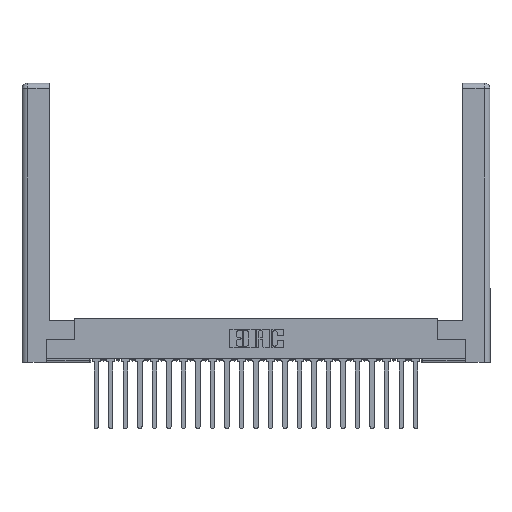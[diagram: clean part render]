
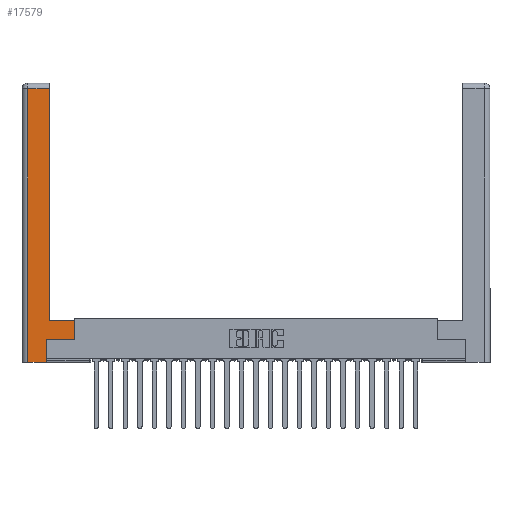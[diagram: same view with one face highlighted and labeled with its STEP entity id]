
A CAD part, top view. The second image highlights one B-rep face of the part: STEP entity #17579.
In plain terms, the highlighted planar face has unit normal (0, 0, 1).
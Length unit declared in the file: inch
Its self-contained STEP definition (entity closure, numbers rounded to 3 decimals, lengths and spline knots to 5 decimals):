
#313 = VERTEX_POINT ( 'NONE', #2295 ) ;
#631 = CARTESIAN_POINT ( 'NONE',  ( 0.265, 0.245, 0. ) ) ;
#657 = VERTEX_POINT ( 'NONE', #1518 ) ;
#1205 = CARTESIAN_POINT ( 'NONE',  ( 0.0615, 2.94, 0. ) ) ;
#1265 = EDGE_CURVE ( 'NONE', #10887, #19889, #2204, .T. ) ;
#1518 = CARTESIAN_POINT ( 'NONE',  ( 0.265, 0., 0. ) ) ;
#1738 = EDGE_CURVE ( 'NONE', #21075, #10887, #23400, .T. ) ;
#1778 = CARTESIAN_POINT ( 'NONE',  ( 0.295, 0.45, 0. ) ) ;
#2204 = LINE ( 'NONE', #16400, #24942 ) ;
#2295 = CARTESIAN_POINT ( 'NONE',  ( 0.265, 0.245, 0. ) ) ;
#2714 = CARTESIAN_POINT ( 'NONE',  ( 0.0615, 2.94, 0. ) ) ;
#4277 = FACE_OUTER_BOUND ( 'NONE', #4990, .T. ) ;
#4420 = ORIENTED_EDGE ( 'NONE', *, *, #1738, .T. ) ;
#4990 = EDGE_LOOP ( 'NONE', ( #19216, #16404, #6336, #10383, #8769, #19691, #4420, #19415 ) ) ;
#5322 = EDGE_CURVE ( 'NONE', #23541, #657, #14976, .T. ) ;
#5569 = CARTESIAN_POINT ( 'NONE',  ( 0.265, 0., 0. ) ) ;
#5839 = VERTEX_POINT ( 'NONE', #9261 ) ;
#5865 = VECTOR ( 'NONE', #8945, 39.37008 ) ;
#5916 = VECTOR ( 'NONE', #13817, 39.37008 ) ;
#6336 = ORIENTED_EDGE ( 'NONE', *, *, #19013, .T. ) ;
#6571 = DIRECTION ( 'NONE',  ( 0., -1., 0. ) ) ;
#7114 = DIRECTION ( 'NONE',  ( -1., 0., 0. ) ) ;
#7325 = LINE ( 'NONE', #16504, #15325 ) ;
#7489 = EDGE_CURVE ( 'NONE', #19889, #5839, #20387, .T. ) ;
#8356 = EDGE_CURVE ( 'NONE', #5839, #15024, #16033, .T. ) ;
#8667 = DIRECTION ( 'NONE',  ( -1., 0., 0. ) ) ;
#8769 = ORIENTED_EDGE ( 'NONE', *, *, #9873, .T. ) ;
#8945 = DIRECTION ( 'NONE',  ( 0., 1., 0. ) ) ;
#9261 = CARTESIAN_POINT ( 'NONE',  ( 0.295, 2.94, 0. ) ) ;
#9380 = DIRECTION ( 'NONE',  ( 1., 0., 0. ) ) ;
#9615 = VECTOR ( 'NONE', #7114, 39.37008 ) ;
#9733 = CARTESIAN_POINT ( 'NONE',  ( 0.0615, 0., 0. ) ) ;
#9873 = EDGE_CURVE ( 'NONE', #657, #313, #15981, .T. ) ;
#10383 = ORIENTED_EDGE ( 'NONE', *, *, #5322, .T. ) ;
#10887 = VERTEX_POINT ( 'NONE', #17751 ) ;
#12091 = CARTESIAN_POINT ( 'NONE',  ( 0.565, 0.245, 0. ) ) ;
#13029 = DIRECTION ( 'NONE',  ( -1., 0., 0. ) ) ;
#13208 = DIRECTION ( 'NONE',  ( 0., 0., -1. ) ) ;
#13454 = VECTOR ( 'NONE', #6571, 39.37008 ) ;
#13817 = DIRECTION ( 'NONE',  ( 0., 1., 0. ) ) ;
#14976 = LINE ( 'NONE', #5569, #17731 ) ;
#15024 = VERTEX_POINT ( 'NONE', #2714 ) ;
#15325 = VECTOR ( 'NONE', #22505, 39.37008 ) ;
#15981 = LINE ( 'NONE', #631, #19985 ) ;
#16033 = LINE ( 'NONE', #1205, #9615 ) ;
#16400 = CARTESIAN_POINT ( 'NONE',  ( 0.295, 0.45, 0. ) ) ;
#16404 = ORIENTED_EDGE ( 'NONE', *, *, #8356, .T. ) ;
#16504 = CARTESIAN_POINT ( 'NONE',  ( 0.565, 0.245, 0. ) ) ;
#17579 = ADVANCED_FACE ( 'NONE', ( #4277 ), #22962, .F. ) ;
#17731 = VECTOR ( 'NONE', #9380, 39.37008 ) ;
#17751 = CARTESIAN_POINT ( 'NONE',  ( 0.565, 0.45, 0. ) ) ;
#18344 = CARTESIAN_POINT ( 'NONE',  ( 0.0615, 0., 0. ) ) ;
#19013 = EDGE_CURVE ( 'NONE', #15024, #23541, #23867, .T. ) ;
#19216 = ORIENTED_EDGE ( 'NONE', *, *, #7489, .T. ) ;
#19415 = ORIENTED_EDGE ( 'NONE', *, *, #1265, .T. ) ;
#19691 = ORIENTED_EDGE ( 'NONE', *, *, #23233, .T. ) ;
#19889 = VERTEX_POINT ( 'NONE', #1778 ) ;
#19985 = VECTOR ( 'NONE', #22092, 39.37008 ) ;
#20387 = LINE ( 'NONE', #25124, #5916 ) ;
#20720 = CARTESIAN_POINT ( 'NONE',  ( 0.565, 0.45, 0. ) ) ;
#21075 = VERTEX_POINT ( 'NONE', #12091 ) ;
#21373 = AXIS2_PLACEMENT_3D ( 'NONE', #22788, #13208, #13029 ) ;
#22092 = DIRECTION ( 'NONE',  ( 0., 1., 0. ) ) ;
#22505 = DIRECTION ( 'NONE',  ( 1., 0., 0. ) ) ;
#22788 = CARTESIAN_POINT ( 'NONE',  ( 0., 0., 0. ) ) ;
#22962 = PLANE ( 'NONE',  #21373 ) ;
#23233 = EDGE_CURVE ( 'NONE', #313, #21075, #7325, .T. ) ;
#23400 = LINE ( 'NONE', #20720, #5865 ) ;
#23541 = VERTEX_POINT ( 'NONE', #9733 ) ;
#23867 = LINE ( 'NONE', #18344, #13454 ) ;
#24942 = VECTOR ( 'NONE', #8667, 39.37008 ) ;
#25124 = CARTESIAN_POINT ( 'NONE',  ( 0.295, 3., 0. ) ) ;
